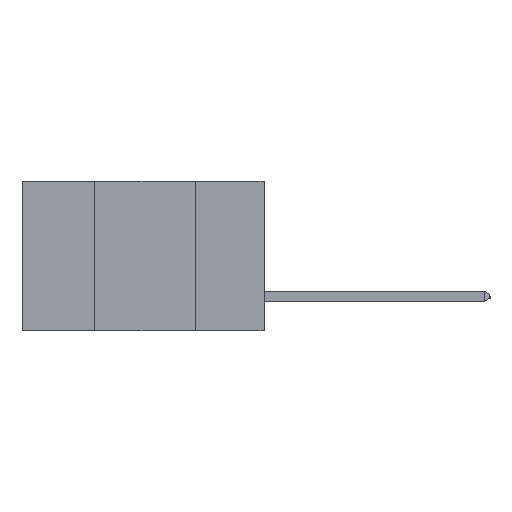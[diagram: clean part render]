
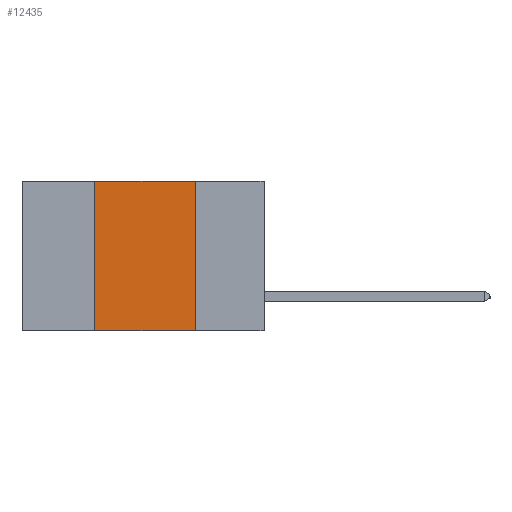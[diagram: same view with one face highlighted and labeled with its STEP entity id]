
A CAD part, left-side view. The second image highlights one B-rep face of the part: STEP entity #12435.
In plain terms, the highlighted planar face has unit normal (-1, 0, 0).
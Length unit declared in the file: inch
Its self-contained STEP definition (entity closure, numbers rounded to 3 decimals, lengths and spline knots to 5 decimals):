
#799 = VERTEX_POINT ( 'NONE', #19576 ) ;
#1191 = DIRECTION ( 'NONE',  ( 0., 0., 1. ) ) ;
#1203 = LINE ( 'NONE', #4506, #14127 ) ;
#2070 = DIRECTION ( 'NONE',  ( 0., -1., 0. ) ) ;
#2226 = ORIENTED_EDGE ( 'NONE', *, *, #8166, .F. ) ;
#3144 = VERTEX_POINT ( 'NONE', #16115 ) ;
#4506 = CARTESIAN_POINT ( 'NONE',  ( 0., 0.42, 0. ) ) ;
#4703 = EDGE_CURVE ( 'NONE', #18842, #3144, #16411, .T. ) ;
#4905 = EDGE_CURVE ( 'NONE', #13460, #799, #20887, .T. ) ;
#5686 = EDGE_LOOP ( 'NONE', ( #2226, #19349, #7058, #11379 ) ) ;
#7058 = ORIENTED_EDGE ( 'NONE', *, *, #17157, .F. ) ;
#7642 = CARTESIAN_POINT ( 'NONE',  ( 0., 0.6, -0.37 ) ) ;
#8166 = EDGE_CURVE ( 'NONE', #3144, #799, #16317, .T. ) ;
#8416 = VECTOR ( 'NONE', #9521, 39.37008 ) ;
#9521 = DIRECTION ( 'NONE',  ( 0., -1., 0. ) ) ;
#9735 = DIRECTION ( 'NONE',  ( 1., 0., 0. ) ) ;
#11379 = ORIENTED_EDGE ( 'NONE', *, *, #4905, .T. ) ;
#11558 = DIRECTION ( 'NONE',  ( 0., 0., -1. ) ) ;
#11573 = CARTESIAN_POINT ( 'NONE',  ( 0., 0.17, 0. ) ) ;
#11614 = VECTOR ( 'NONE', #11558, 39.37008 ) ;
#11934 = FACE_OUTER_BOUND ( 'NONE', #5686, .T. ) ;
#12435 = ADVANCED_FACE ( 'NONE', ( #11934 ), #19300, .F. ) ;
#13460 = VERTEX_POINT ( 'NONE', #20572 ) ;
#14127 = VECTOR ( 'NONE', #1191, 39.37008 ) ;
#16071 = CARTESIAN_POINT ( 'NONE',  ( 0., 0.6, 0. ) ) ;
#16115 = CARTESIAN_POINT ( 'NONE',  ( 0., 0.17, 0. ) ) ;
#16317 = LINE ( 'NONE', #11573, #11614 ) ;
#16411 = LINE ( 'NONE', #17263, #8416 ) ;
#17157 = EDGE_CURVE ( 'NONE', #13460, #18842, #1203, .T. ) ;
#17168 = VECTOR ( 'NONE', #2070, 39.37008 ) ;
#17263 = CARTESIAN_POINT ( 'NONE',  ( 0., 0.6, 0. ) ) ;
#18842 = VERTEX_POINT ( 'NONE', #19113 ) ;
#19080 = AXIS2_PLACEMENT_3D ( 'NONE', #16071, #9735, #20888 ) ;
#19113 = CARTESIAN_POINT ( 'NONE',  ( 0., 0.42, 0. ) ) ;
#19300 = PLANE ( 'NONE',  #19080 ) ;
#19349 = ORIENTED_EDGE ( 'NONE', *, *, #4703, .F. ) ;
#19576 = CARTESIAN_POINT ( 'NONE',  ( 0., 0.17, -0.37 ) ) ;
#20572 = CARTESIAN_POINT ( 'NONE',  ( 0., 0.42, -0.37 ) ) ;
#20887 = LINE ( 'NONE', #7642, #17168 ) ;
#20888 = DIRECTION ( 'NONE',  ( 0., 0., -1. ) ) ;
